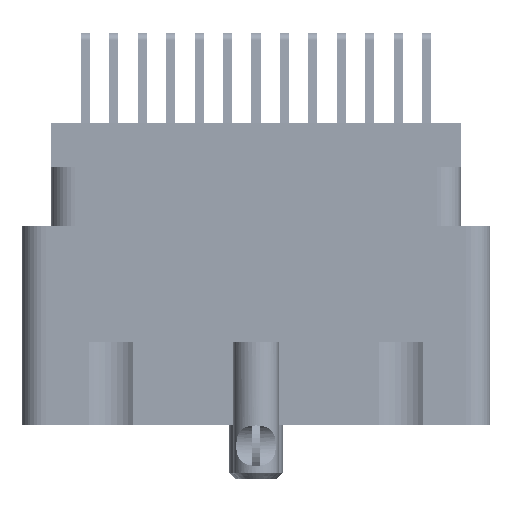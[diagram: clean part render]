
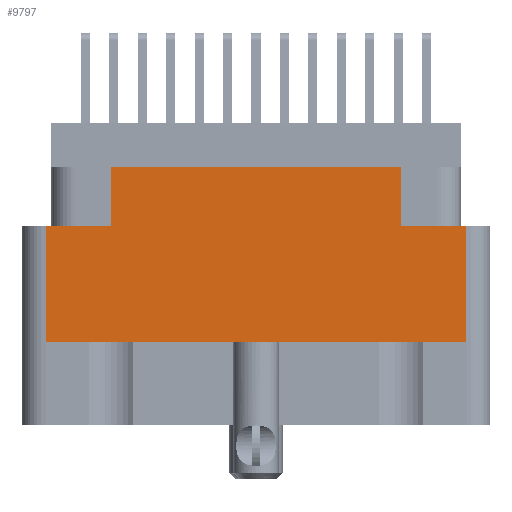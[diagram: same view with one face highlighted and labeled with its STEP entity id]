
A CAD part, left-side view. The second image highlights one B-rep face of the part: STEP entity #9797.
In plain terms, the highlighted planar face has unit normal (-1, 0, 0).
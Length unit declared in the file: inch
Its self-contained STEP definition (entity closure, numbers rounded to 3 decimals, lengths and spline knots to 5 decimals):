
#1710 = VECTOR ( 'NONE', #75038, 39.37008 ) ;
#5220 = ORIENTED_EDGE ( 'NONE', *, *, #24726, .T. ) ;
#6082 = VERTEX_POINT ( 'NONE', #30592 ) ;
#7557 = EDGE_CURVE ( 'NONE', #59263, #37465, #51678, .T. ) ;
#8692 = VECTOR ( 'NONE', #76468, 39.37008 ) ;
#9197 = VERTEX_POINT ( 'NONE', #79352 ) ;
#9797 = ADVANCED_FACE ( 'NONE', ( #77606 ), #65427, .T. ) ;
#10438 = CARTESIAN_POINT ( 'NONE',  ( -1.359, -0.3825, -0.274 ) ) ;
#11394 = DIRECTION ( 'NONE',  ( 0., 0., 1. ) ) ;
#14683 = ORIENTED_EDGE ( 'NONE', *, *, #29457, .T. ) ;
#15823 = VERTEX_POINT ( 'NONE', #30593 ) ;
#18613 = LINE ( 'NONE', #30094, #66052 ) ;
#19456 = CARTESIAN_POINT ( 'NONE',  ( -1.359, -0.555, -0.274 ) ) ;
#22816 = EDGE_CURVE ( 'NONE', #37465, #6082, #65526, .T. ) ;
#24337 = DIRECTION ( 'NONE',  ( 0., -1., 0. ) ) ;
#24726 = EDGE_CURVE ( 'NONE', #15823, #6082, #39150, .T. ) ;
#25720 = LINE ( 'NONE', #66007, #70154 ) ;
#26060 = CARTESIAN_POINT ( 'NONE',  ( -1.359, 0., -0.578 ) ) ;
#26330 = VECTOR ( 'NONE', #80499, 39.37008 ) ;
#26940 = EDGE_CURVE ( 'NONE', #15823, #41989, #60631, .T. ) ;
#28137 = DIRECTION ( 'NONE',  ( 0., 0., 1. ) ) ;
#28564 = CARTESIAN_POINT ( 'NONE',  ( -1.359, 0.3825, -0.117 ) ) ;
#29457 = EDGE_CURVE ( 'NONE', #74675, #41989, #25720, .T. ) ;
#30094 = CARTESIAN_POINT ( 'NONE',  ( -1.359, 0., -0.274 ) ) ;
#30592 = CARTESIAN_POINT ( 'NONE',  ( -1.359, -0.3825, -0.117 ) ) ;
#30593 = CARTESIAN_POINT ( 'NONE',  ( -1.359, -0.3825, -0.274 ) ) ;
#30857 = CARTESIAN_POINT ( 'NONE',  ( -1.359, 0., -0.274 ) ) ;
#32234 = CARTESIAN_POINT ( 'NONE',  ( -1.359, -0.617, -0.798 ) ) ;
#33080 = ORIENTED_EDGE ( 'NONE', *, *, #26940, .F. ) ;
#37465 = VERTEX_POINT ( 'NONE', #28564 ) ;
#39150 = LINE ( 'NONE', #10438, #26330 ) ;
#39159 = CARTESIAN_POINT ( 'NONE',  ( -1.359, 0.617, -0.117 ) ) ;
#39864 = CARTESIAN_POINT ( 'NONE',  ( -1.359, -0.555, -0.578 ) ) ;
#41400 = EDGE_CURVE ( 'NONE', #68204, #74675, #75784, .T. ) ;
#41616 = EDGE_CURVE ( 'NONE', #9197, #68204, #59997, .T. ) ;
#41989 = VERTEX_POINT ( 'NONE', #19456 ) ;
#42696 = ORIENTED_EDGE ( 'NONE', *, *, #65667, .F. ) ;
#48861 = CARTESIAN_POINT ( 'NONE',  ( -1.359, 0.555, -0.578 ) ) ;
#49908 = DIRECTION ( 'NONE',  ( 0., -1., 0. ) ) ;
#50523 = ORIENTED_EDGE ( 'NONE', *, *, #41616, .T. ) ;
#51211 = ORIENTED_EDGE ( 'NONE', *, *, #22816, .F. ) ;
#51678 = LINE ( 'NONE', #73700, #56627 ) ;
#56627 = VECTOR ( 'NONE', #11394, 39.37008 ) ;
#56836 = DIRECTION ( 'NONE',  ( -1., 0., 0. ) ) ;
#57018 = EDGE_LOOP ( 'NONE', ( #42696, #50523, #68332, #14683, #33080, #5220, #51211, #78379 ) ) ;
#57554 = VECTOR ( 'NONE', #59275, 39.37008 ) ;
#59263 = VERTEX_POINT ( 'NONE', #69233 ) ;
#59275 = DIRECTION ( 'NONE',  ( 0., -1., 0. ) ) ;
#59997 = LINE ( 'NONE', #62152, #1710 ) ;
#60631 = LINE ( 'NONE', #30857, #68590 ) ;
#62152 = CARTESIAN_POINT ( 'NONE',  ( -1.359, 0.555, -0.798 ) ) ;
#65427 = PLANE ( 'NONE',  #75634 ) ;
#65526 = LINE ( 'NONE', #39159, #57554 ) ;
#65667 = EDGE_CURVE ( 'NONE', #9197, #59263, #18613, .T. ) ;
#66007 = CARTESIAN_POINT ( 'NONE',  ( -1.359, -0.555, -0.798 ) ) ;
#66052 = VECTOR ( 'NONE', #24337, 39.37008 ) ;
#68204 = VERTEX_POINT ( 'NONE', #48861 ) ;
#68332 = ORIENTED_EDGE ( 'NONE', *, *, #41400, .T. ) ;
#68590 = VECTOR ( 'NONE', #49908, 39.37008 ) ;
#69233 = CARTESIAN_POINT ( 'NONE',  ( -1.359, 0.3825, -0.274 ) ) ;
#70154 = VECTOR ( 'NONE', #28137, 39.37008 ) ;
#73700 = CARTESIAN_POINT ( 'NONE',  ( -1.359, 0.3825, -0.274 ) ) ;
#74675 = VERTEX_POINT ( 'NONE', #39864 ) ;
#75038 = DIRECTION ( 'NONE',  ( 0., 0., -1. ) ) ;
#75634 = AXIS2_PLACEMENT_3D ( 'NONE', #32234, #56836, #77750 ) ;
#75784 = LINE ( 'NONE', #26060, #8692 ) ;
#76468 = DIRECTION ( 'NONE',  ( 0., -1., 0. ) ) ;
#77606 = FACE_OUTER_BOUND ( 'NONE', #57018, .T. ) ;
#77750 = DIRECTION ( 'NONE',  ( 0., 0., 1. ) ) ;
#78379 = ORIENTED_EDGE ( 'NONE', *, *, #7557, .F. ) ;
#79352 = CARTESIAN_POINT ( 'NONE',  ( -1.359, 0.555, -0.274 ) ) ;
#80499 = DIRECTION ( 'NONE',  ( 0., 0., 1. ) ) ;
